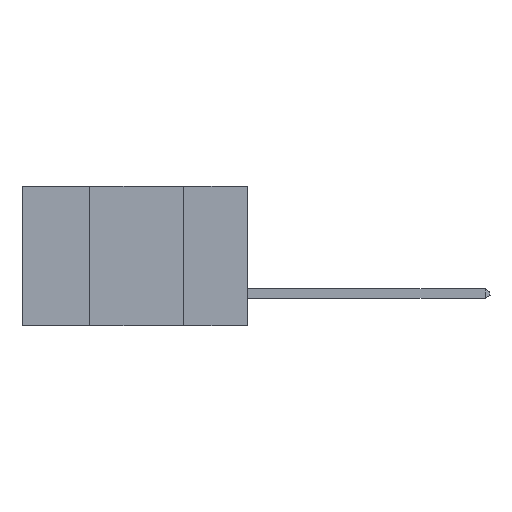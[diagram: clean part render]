
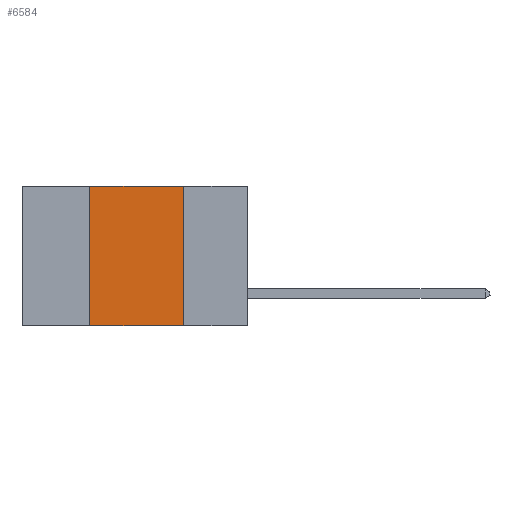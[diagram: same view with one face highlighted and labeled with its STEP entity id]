
A CAD part, left-side view. The second image highlights one B-rep face of the part: STEP entity #6584.
In plain terms, the highlighted planar face has unit normal (-1, 0, 0).
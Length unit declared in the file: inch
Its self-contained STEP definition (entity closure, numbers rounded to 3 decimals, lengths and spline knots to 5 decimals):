
#173 = DIRECTION ( 'NONE',  ( 1., 0., 0. ) ) ;
#920 = LINE ( 'NONE', #18430, #14411 ) ;
#1032 = AXIS2_PLACEMENT_3D ( 'NONE', #21046, #173, #21344 ) ;
#1498 = EDGE_CURVE ( 'NONE', #29016, #11526, #4357, .T. ) ;
#1691 = EDGE_LOOP ( 'NONE', ( #12725, #18336, #29432, #4820 ) ) ;
#1767 = DIRECTION ( 'NONE',  ( 0., 0., 1. ) ) ;
#2784 = CARTESIAN_POINT ( 'NONE',  ( 0., 0.6, -0.37 ) ) ;
#4357 = LINE ( 'NONE', #22627, #14881 ) ;
#4564 = VERTEX_POINT ( 'NONE', #8438 ) ;
#4820 = ORIENTED_EDGE ( 'NONE', *, *, #4831, .T. ) ;
#4831 = EDGE_CURVE ( 'NONE', #29016, #4564, #12684, .T. ) ;
#6391 = EDGE_CURVE ( 'NONE', #14323, #4564, #14979, .T. ) ;
#6584 = ADVANCED_FACE ( 'NONE', ( #14187 ), #9922, .F. ) ;
#7826 = CARTESIAN_POINT ( 'NONE',  ( 0., 0.42, -0.37 ) ) ;
#7957 = DIRECTION ( 'NONE',  ( 0., -1., 0. ) ) ;
#8109 = EDGE_CURVE ( 'NONE', #11526, #14323, #920, .T. ) ;
#8438 = CARTESIAN_POINT ( 'NONE',  ( 0., 0.17, -0.37 ) ) ;
#9922 = PLANE ( 'NONE',  #1032 ) ;
#11150 = CARTESIAN_POINT ( 'NONE',  ( 0., 0.17, 0. ) ) ;
#11526 = VERTEX_POINT ( 'NONE', #22074 ) ;
#12672 = VECTOR ( 'NONE', #15874, 39.37008 ) ;
#12684 = LINE ( 'NONE', #2784, #18389 ) ;
#12725 = ORIENTED_EDGE ( 'NONE', *, *, #6391, .F. ) ;
#14187 = FACE_OUTER_BOUND ( 'NONE', #1691, .T. ) ;
#14323 = VERTEX_POINT ( 'NONE', #20748 ) ;
#14411 = VECTOR ( 'NONE', #22835, 39.37008 ) ;
#14881 = VECTOR ( 'NONE', #1767, 39.37008 ) ;
#14979 = LINE ( 'NONE', #11150, #12672 ) ;
#15874 = DIRECTION ( 'NONE',  ( 0., 0., -1. ) ) ;
#18336 = ORIENTED_EDGE ( 'NONE', *, *, #8109, .F. ) ;
#18389 = VECTOR ( 'NONE', #7957, 39.37008 ) ;
#18430 = CARTESIAN_POINT ( 'NONE',  ( 0., 0.6, 0. ) ) ;
#20748 = CARTESIAN_POINT ( 'NONE',  ( 0., 0.17, 0. ) ) ;
#21046 = CARTESIAN_POINT ( 'NONE',  ( 0., 0.6, 0. ) ) ;
#21344 = DIRECTION ( 'NONE',  ( 0., 0., -1. ) ) ;
#22074 = CARTESIAN_POINT ( 'NONE',  ( 0., 0.42, 0. ) ) ;
#22627 = CARTESIAN_POINT ( 'NONE',  ( 0., 0.42, 0. ) ) ;
#22835 = DIRECTION ( 'NONE',  ( 0., -1., 0. ) ) ;
#29016 = VERTEX_POINT ( 'NONE', #7826 ) ;
#29432 = ORIENTED_EDGE ( 'NONE', *, *, #1498, .F. ) ;
